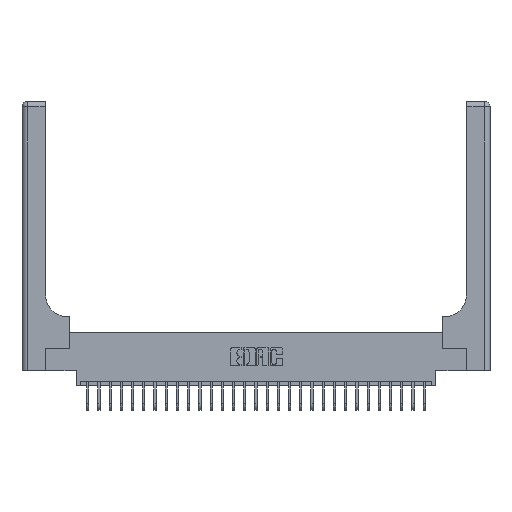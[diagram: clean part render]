
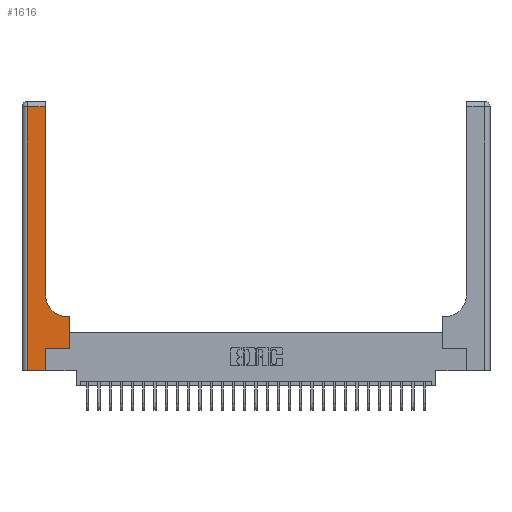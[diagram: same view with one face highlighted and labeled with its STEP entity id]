
A CAD part, top view. The second image highlights one B-rep face of the part: STEP entity #1616.
In plain terms, the highlighted planar face has unit normal (0, 0, 1).
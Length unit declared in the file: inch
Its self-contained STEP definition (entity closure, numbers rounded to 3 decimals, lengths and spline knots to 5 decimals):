
#33 = CARTESIAN_POINT ( 'NONE',  ( 0.528, 0.6, 0.37 ) ) ;
#304 = CARTESIAN_POINT ( 'NONE',  ( 0.265, 0., 0.37 ) ) ;
#358 = CARTESIAN_POINT ( 'NONE',  ( 0.26, 3., 0.37 ) ) ;
#675 = EDGE_CURVE ( 'NONE', #14712, #24085, #21765, .T. ) ;
#914 = DIRECTION ( 'NONE',  ( 0., 0., -1. ) ) ;
#1044 = EDGE_CURVE ( 'NONE', #7909, #6910, #2879, .T. ) ;
#1616 = ADVANCED_FACE ( 'NONE', ( #15045 ), #17049, .F. ) ;
#2282 = VERTEX_POINT ( 'NONE', #11541 ) ;
#2795 = CARTESIAN_POINT ( 'NONE',  ( 0., 0., 0.37 ) ) ;
#2879 = CIRCLE ( 'NONE', #21778, 0.25 ) ;
#3188 = EDGE_CURVE ( 'NONE', #4095, #2282, #4882, .T. ) ;
#3454 = VECTOR ( 'NONE', #21104, 39.37008 ) ;
#3511 = CARTESIAN_POINT ( 'NONE',  ( 0.265, 0.25, 0.37 ) ) ;
#4095 = VERTEX_POINT ( 'NONE', #5580 ) ;
#4657 = CARTESIAN_POINT ( 'NONE',  ( 0.265, 0., 0.37 ) ) ;
#4882 = LINE ( 'NONE', #3511, #18830 ) ;
#4946 = CARTESIAN_POINT ( 'NONE',  ( 0.26, 0.6, 0.37 ) ) ;
#5284 = EDGE_CURVE ( 'NONE', #2282, #17497, #16042, .T. ) ;
#5358 = LINE ( 'NONE', #4946, #26120 ) ;
#5580 = CARTESIAN_POINT ( 'NONE',  ( 0.265, 0.25, 0.37 ) ) ;
#5849 = CARTESIAN_POINT ( 'NONE',  ( 0.528, 0.25, 0.37 ) ) ;
#6275 = LINE ( 'NONE', #4657, #6976 ) ;
#6313 = VECTOR ( 'NONE', #24960, 39.37008 ) ;
#6660 = ORIENTED_EDGE ( 'NONE', *, *, #675, .T. ) ;
#6910 = VERTEX_POINT ( 'NONE', #18181 ) ;
#6976 = VECTOR ( 'NONE', #12718, 39.37008 ) ;
#7611 = AXIS2_PLACEMENT_3D ( 'NONE', #23393, #21110, #12768 ) ;
#7667 = DIRECTION ( 'NONE',  ( 1., 0., 0. ) ) ;
#7909 = VERTEX_POINT ( 'NONE', #18908 ) ;
#9240 = DIRECTION ( 'NONE',  ( 1., 0., 0. ) ) ;
#9728 = ORIENTED_EDGE ( 'NONE', *, *, #3188, .T. ) ;
#9791 = CARTESIAN_POINT ( 'NONE',  ( 0., 2.94, 0.37 ) ) ;
#10184 = EDGE_CURVE ( 'NONE', #24085, #15041, #20963, .T. ) ;
#11000 = ORIENTED_EDGE ( 'NONE', *, *, #5284, .T. ) ;
#11538 = ORIENTED_EDGE ( 'NONE', *, *, #17822, .T. ) ;
#11541 = CARTESIAN_POINT ( 'NONE',  ( 0.528, 0.25, 0.37 ) ) ;
#12718 = DIRECTION ( 'NONE',  ( 0., 1., 0. ) ) ;
#12768 = DIRECTION ( 'NONE',  ( -1., 0., 0. ) ) ;
#12816 = EDGE_CURVE ( 'NONE', #6910, #14712, #18761, .T. ) ;
#13149 = VECTOR ( 'NONE', #24188, 39.37008 ) ;
#14084 = EDGE_CURVE ( 'NONE', #15041, #14866, #14995, .T. ) ;
#14712 = VERTEX_POINT ( 'NONE', #23975 ) ;
#14866 = VERTEX_POINT ( 'NONE', #304 ) ;
#14995 = LINE ( 'NONE', #2795, #6313 ) ;
#15029 = ORIENTED_EDGE ( 'NONE', *, *, #1044, .T. ) ;
#15041 = VERTEX_POINT ( 'NONE', #22432 ) ;
#15045 = FACE_OUTER_BOUND ( 'NONE', #23590, .T. ) ;
#16042 = LINE ( 'NONE', #5849, #16273 ) ;
#16273 = VECTOR ( 'NONE', #24389, 39.37008 ) ;
#16583 = CARTESIAN_POINT ( 'NONE',  ( 0.06, 2.94, 0.37 ) ) ;
#16729 = DIRECTION ( 'NONE',  ( 0., 1., 0. ) ) ;
#17049 = PLANE ( 'NONE',  #7611 ) ;
#17497 = VERTEX_POINT ( 'NONE', #33 ) ;
#17529 = EDGE_CURVE ( 'NONE', #17497, #7909, #5358, .T. ) ;
#17822 = EDGE_CURVE ( 'NONE', #14866, #4095, #6275, .T. ) ;
#18181 = CARTESIAN_POINT ( 'NONE',  ( 0.26, 0.85, 0.37 ) ) ;
#18761 = LINE ( 'NONE', #358, #24457 ) ;
#18830 = VECTOR ( 'NONE', #7667, 39.37008 ) ;
#18908 = CARTESIAN_POINT ( 'NONE',  ( 0.51, 0.6, 0.37 ) ) ;
#20503 = ORIENTED_EDGE ( 'NONE', *, *, #14084, .T. ) ;
#20963 = LINE ( 'NONE', #25138, #3454 ) ;
#21104 = DIRECTION ( 'NONE',  ( 0., -1., 0. ) ) ;
#21110 = DIRECTION ( 'NONE',  ( 0., 0., -1. ) ) ;
#21618 = CARTESIAN_POINT ( 'NONE',  ( 0.51, 0.85, 0.37 ) ) ;
#21635 = DIRECTION ( 'NONE',  ( -1., 0., 0. ) ) ;
#21765 = LINE ( 'NONE', #9791, #13149 ) ;
#21778 = AXIS2_PLACEMENT_3D ( 'NONE', #21618, #914, #9240 ) ;
#22327 = ORIENTED_EDGE ( 'NONE', *, *, #12816, .T. ) ;
#22432 = CARTESIAN_POINT ( 'NONE',  ( 0.06, 0., 0.37 ) ) ;
#22988 = ORIENTED_EDGE ( 'NONE', *, *, #17529, .T. ) ;
#23393 = CARTESIAN_POINT ( 'NONE',  ( 0., 3., 0.37 ) ) ;
#23590 = EDGE_LOOP ( 'NONE', ( #22327, #6660, #25489, #20503, #11538, #9728, #11000, #22988, #15029 ) ) ;
#23975 = CARTESIAN_POINT ( 'NONE',  ( 0.26, 2.94, 0.37 ) ) ;
#24085 = VERTEX_POINT ( 'NONE', #16583 ) ;
#24188 = DIRECTION ( 'NONE',  ( -1., 0., 0. ) ) ;
#24389 = DIRECTION ( 'NONE',  ( 0., 1., 0. ) ) ;
#24457 = VECTOR ( 'NONE', #16729, 39.37008 ) ;
#24960 = DIRECTION ( 'NONE',  ( 1., 0., 0. ) ) ;
#25138 = CARTESIAN_POINT ( 'NONE',  ( 0.06, 3., 0.37 ) ) ;
#25489 = ORIENTED_EDGE ( 'NONE', *, *, #10184, .T. ) ;
#26120 = VECTOR ( 'NONE', #21635, 39.37008 ) ;
